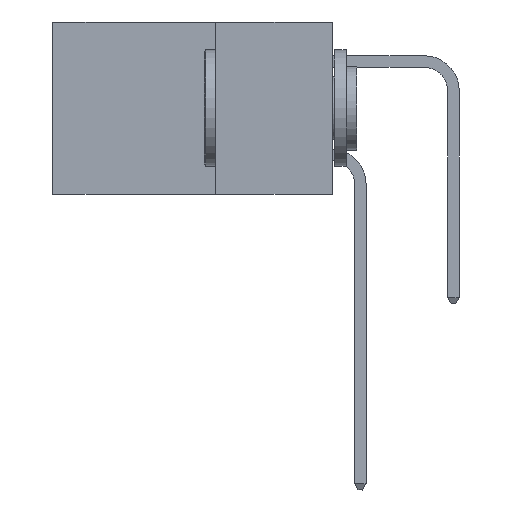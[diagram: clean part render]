
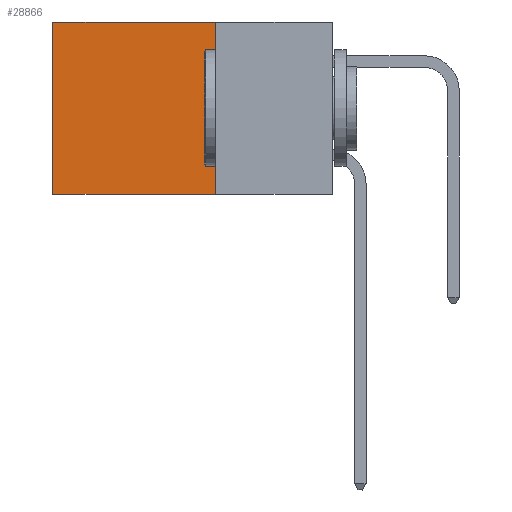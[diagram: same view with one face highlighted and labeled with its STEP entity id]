
A CAD part, left-side view. The second image highlights one B-rep face of the part: STEP entity #28866.
In plain terms, the highlighted planar face has unit normal (-1, 0, 0).
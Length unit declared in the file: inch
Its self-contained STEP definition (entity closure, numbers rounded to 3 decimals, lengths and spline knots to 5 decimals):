
#281 = CARTESIAN_POINT ( 'NONE',  ( 0.2615, 0.25, 0. ) ) ;
#1294 = CARTESIAN_POINT ( 'NONE',  ( 0.2615, 0.25, -0.37 ) ) ;
#1588 = DIRECTION ( 'NONE',  ( 0., 0., -1. ) ) ;
#1645 = DIRECTION ( 'NONE',  ( 0., 1., 0. ) ) ;
#2342 = EDGE_LOOP ( 'NONE', ( #5893, #24703, #12493, #12451 ) ) ;
#3491 = LINE ( 'NONE', #12618, #25290 ) ;
#5893 = ORIENTED_EDGE ( 'NONE', *, *, #29304, .T. ) ;
#5912 = DIRECTION ( 'NONE',  ( 0., 0., -1. ) ) ;
#6118 = VERTEX_POINT ( 'NONE', #8777 ) ;
#8124 = DIRECTION ( 'NONE',  ( 0., 0., -1. ) ) ;
#8154 = DIRECTION ( 'NONE',  ( 1., 0., 0. ) ) ;
#8777 = CARTESIAN_POINT ( 'NONE',  ( 0.2615, 0.6, 0. ) ) ;
#12451 = ORIENTED_EDGE ( 'NONE', *, *, #19156, .T. ) ;
#12493 = ORIENTED_EDGE ( 'NONE', *, *, #25676, .F. ) ;
#12618 = CARTESIAN_POINT ( 'NONE',  ( 0.2615, 0.6, -0.37 ) ) ;
#15999 = CARTESIAN_POINT ( 'NONE',  ( 0.2615, 0.25, 0. ) ) ;
#16674 = VERTEX_POINT ( 'NONE', #281 ) ;
#17235 = VERTEX_POINT ( 'NONE', #23372 ) ;
#17455 = VECTOR ( 'NONE', #1645, 39.37008 ) ;
#18362 = EDGE_CURVE ( 'NONE', #17235, #22406, #20319, .T. ) ;
#19156 = EDGE_CURVE ( 'NONE', #16674, #6118, #27492, .T. ) ;
#20111 = LINE ( 'NONE', #22053, #26648 ) ;
#20319 = LINE ( 'NONE', #24328, #17455 ) ;
#20656 = DIRECTION ( 'NONE',  ( 0., 1., 0. ) ) ;
#20847 = VECTOR ( 'NONE', #20656, 39.37008 ) ;
#21770 = PLANE ( 'NONE',  #26215 ) ;
#21918 = FACE_OUTER_BOUND ( 'NONE', #2342, .T. ) ;
#22053 = CARTESIAN_POINT ( 'NONE',  ( 0.2615, 0.25, -0.37 ) ) ;
#22406 = VERTEX_POINT ( 'NONE', #27255 ) ;
#23372 = CARTESIAN_POINT ( 'NONE',  ( 0.2615, 0.25, -0.37 ) ) ;
#24328 = CARTESIAN_POINT ( 'NONE',  ( 0.2615, 0.25, -0.37 ) ) ;
#24703 = ORIENTED_EDGE ( 'NONE', *, *, #18362, .F. ) ;
#25290 = VECTOR ( 'NONE', #8124, 39.37008 ) ;
#25676 = EDGE_CURVE ( 'NONE', #16674, #17235, #20111, .T. ) ;
#26215 = AXIS2_PLACEMENT_3D ( 'NONE', #1294, #8154, #5912 ) ;
#26648 = VECTOR ( 'NONE', #1588, 39.37008 ) ;
#27255 = CARTESIAN_POINT ( 'NONE',  ( 0.2615, 0.6, -0.37 ) ) ;
#27492 = LINE ( 'NONE', #15999, #20847 ) ;
#28866 = ADVANCED_FACE ( 'NONE', ( #21918 ), #21770, .F. ) ;
#29304 = EDGE_CURVE ( 'NONE', #6118, #22406, #3491, .T. ) ;
